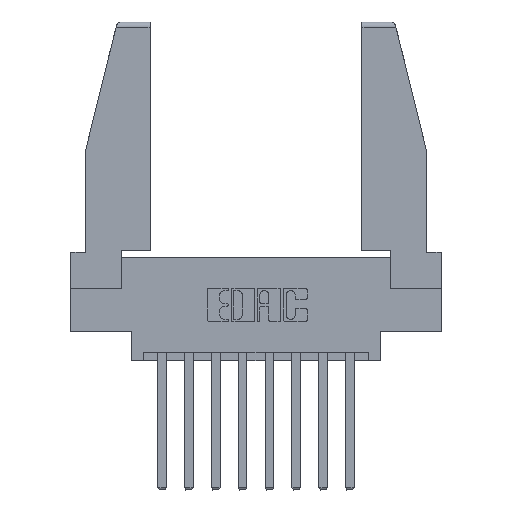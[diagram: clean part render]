
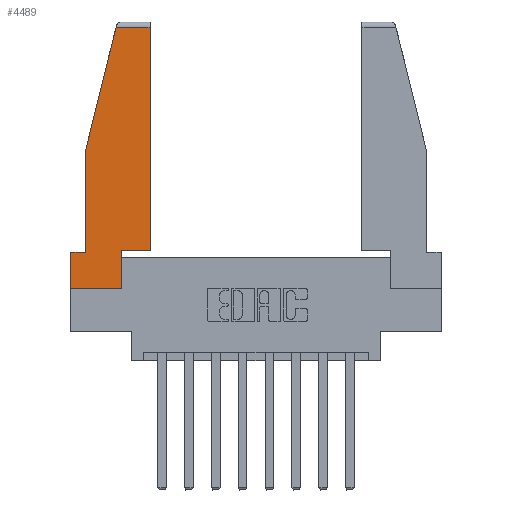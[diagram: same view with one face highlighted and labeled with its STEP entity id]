
A CAD part, top view. The second image highlights one B-rep face of the part: STEP entity #4489.
In plain terms, the highlighted planar face has unit normal (0, 0, 1).
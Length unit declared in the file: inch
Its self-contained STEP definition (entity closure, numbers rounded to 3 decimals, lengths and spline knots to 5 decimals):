
#31 = CARTESIAN_POINT ( 'NONE',  ( 0.461, 1.52, 0. ) ) ;
#42 = FACE_OUTER_BOUND ( 'NONE', #4486, .T. ) ;
#268 = EDGE_CURVE ( 'NONE', #4626, #12606, #3107, .T. ) ;
#303 = CARTESIAN_POINT ( 'NONE',  ( 0.461, 0.223, 0. ) ) ;
#670 = CARTESIAN_POINT ( 'NONE',  ( 0., 0.21, 0. ) ) ;
#690 = VERTEX_POINT ( 'NONE', #11882 ) ;
#905 = EDGE_CURVE ( 'NONE', #12606, #11230, #9259, .T. ) ;
#921 = CARTESIAN_POINT ( 'NONE',  ( 0.271, 1.55, 0. ) ) ;
#1082 = DIRECTION ( 'NONE',  ( 0., 0., 1. ) ) ;
#1166 = ORIENTED_EDGE ( 'NONE', *, *, #2799, .T. ) ;
#1226 = CARTESIAN_POINT ( 'NONE',  ( 0., 0., 0. ) ) ;
#1301 = LINE ( 'NONE', #2824, #9326 ) ;
#1566 = ORIENTED_EDGE ( 'NONE', *, *, #12931, .T. ) ;
#1615 = VECTOR ( 'NONE', #2732, 39.37008 ) ;
#1993 = CARTESIAN_POINT ( 'NONE',  ( 0.297, 0., 0. ) ) ;
#2025 = DIRECTION ( 'NONE',  ( 0., 1., 0. ) ) ;
#2594 = CARTESIAN_POINT ( 'NONE',  ( 0.461, 0.223, 0. ) ) ;
#2602 = LINE ( 'NONE', #921, #10327 ) ;
#2680 = AXIS2_PLACEMENT_3D ( 'NONE', #1226, #1082, #10290 ) ;
#2732 = DIRECTION ( 'NONE',  ( -1., 0., 0. ) ) ;
#2799 = EDGE_CURVE ( 'NONE', #10244, #4626, #2602, .T. ) ;
#2824 = CARTESIAN_POINT ( 'NONE',  ( 0., 0.21, 0. ) ) ;
#3025 = VERTEX_POINT ( 'NONE', #2594 ) ;
#3057 = CARTESIAN_POINT ( 'NONE',  ( 0.297, 0.223, 0. ) ) ;
#3107 = LINE ( 'NONE', #7258, #11778 ) ;
#3350 = VECTOR ( 'NONE', #8898, 39.37008 ) ;
#3354 = CARTESIAN_POINT ( 'NONE',  ( 0., 0., 0. ) ) ;
#3681 = ORIENTED_EDGE ( 'NONE', *, *, #11573, .T. ) ;
#3820 = ORIENTED_EDGE ( 'NONE', *, *, #268, .T. ) ;
#3913 = CARTESIAN_POINT ( 'NONE',  ( 0., 1.52, 0. ) ) ;
#4004 = DIRECTION ( 'NONE',  ( -0.239, -0.971, 0. ) ) ;
#4126 = ORIENTED_EDGE ( 'NONE', *, *, #4143, .T. ) ;
#4143 = EDGE_CURVE ( 'NONE', #7692, #10244, #9796, .T. ) ;
#4440 = CARTESIAN_POINT ( 'NONE',  ( 0.086, 0.8, 0. ) ) ;
#4486 = EDGE_LOOP ( 'NONE', ( #10350, #4126, #1166, #3820, #11920, #3681, #1566, #5857, #10539 ) ) ;
#4489 = ADVANCED_FACE ( 'NONE', ( #42 ), #6241, .T. ) ;
#4626 = VERTEX_POINT ( 'NONE', #4440 ) ;
#4953 = EDGE_CURVE ( 'NONE', #690, #3025, #5545, .T. ) ;
#5383 = LINE ( 'NONE', #9973, #11013 ) ;
#5545 = LINE ( 'NONE', #3057, #7119 ) ;
#5857 = ORIENTED_EDGE ( 'NONE', *, *, #6498, .T. ) ;
#6241 = PLANE ( 'NONE',  #2680 ) ;
#6498 = EDGE_CURVE ( 'NONE', #8566, #690, #5383, .T. ) ;
#6724 = VERTEX_POINT ( 'NONE', #3354 ) ;
#6900 = EDGE_CURVE ( 'NONE', #3025, #7692, #11316, .T. ) ;
#6919 = VECTOR ( 'NONE', #2025, 39.37008 ) ;
#7119 = VECTOR ( 'NONE', #9339, 39.37008 ) ;
#7258 = CARTESIAN_POINT ( 'NONE',  ( 0.086, 0.8, 0. ) ) ;
#7302 = CARTESIAN_POINT ( 'NONE',  ( 0., 0.21, 0. ) ) ;
#7692 = VERTEX_POINT ( 'NONE', #31 ) ;
#8069 = CARTESIAN_POINT ( 'NONE',  ( 0.2636, 1.52, 0. ) ) ;
#8566 = VERTEX_POINT ( 'NONE', #1993 ) ;
#8628 = DIRECTION ( 'NONE',  ( -1., 0., 0. ) ) ;
#8834 = DIRECTION ( 'NONE',  ( 0., -1., 0. ) ) ;
#8898 = DIRECTION ( 'NONE',  ( 1., 0., 0. ) ) ;
#9259 = LINE ( 'NONE', #670, #12564 ) ;
#9326 = VECTOR ( 'NONE', #8834, 39.37008 ) ;
#9339 = DIRECTION ( 'NONE',  ( 1., 0., 0. ) ) ;
#9665 = DIRECTION ( 'NONE',  ( 0., -1., 0. ) ) ;
#9796 = LINE ( 'NONE', #3913, #1615 ) ;
#9973 = CARTESIAN_POINT ( 'NONE',  ( 0.297, 0., 0. ) ) ;
#10244 = VERTEX_POINT ( 'NONE', #8069 ) ;
#10290 = DIRECTION ( 'NONE',  ( 1., 0., 0. ) ) ;
#10327 = VECTOR ( 'NONE', #4004, 39.37008 ) ;
#10350 = ORIENTED_EDGE ( 'NONE', *, *, #6900, .T. ) ;
#10539 = ORIENTED_EDGE ( 'NONE', *, *, #4953, .T. ) ;
#11013 = VECTOR ( 'NONE', #12002, 39.37008 ) ;
#11230 = VERTEX_POINT ( 'NONE', #7302 ) ;
#11316 = LINE ( 'NONE', #303, #6919 ) ;
#11356 = LINE ( 'NONE', #11897, #3350 ) ;
#11573 = EDGE_CURVE ( 'NONE', #11230, #6724, #1301, .T. ) ;
#11778 = VECTOR ( 'NONE', #9665, 39.37008 ) ;
#11882 = CARTESIAN_POINT ( 'NONE',  ( 0.297, 0.223, 0. ) ) ;
#11897 = CARTESIAN_POINT ( 'NONE',  ( 0., 0., 0. ) ) ;
#11920 = ORIENTED_EDGE ( 'NONE', *, *, #905, .T. ) ;
#12002 = DIRECTION ( 'NONE',  ( 0., 1., 0. ) ) ;
#12564 = VECTOR ( 'NONE', #8628, 39.37008 ) ;
#12606 = VERTEX_POINT ( 'NONE', #12713 ) ;
#12713 = CARTESIAN_POINT ( 'NONE',  ( 0.086, 0.21, 0. ) ) ;
#12931 = EDGE_CURVE ( 'NONE', #6724, #8566, #11356, .T. ) ;
